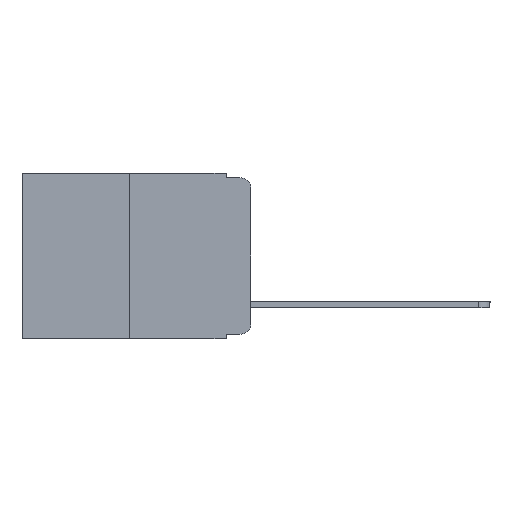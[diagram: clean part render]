
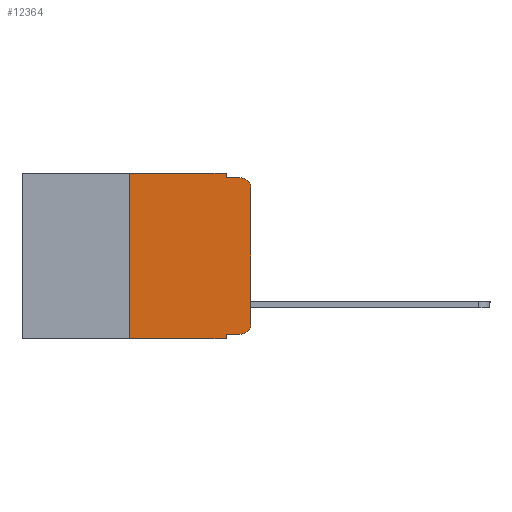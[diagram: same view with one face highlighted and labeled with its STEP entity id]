
A CAD part, left-side view. The second image highlights one B-rep face of the part: STEP entity #12364.
In plain terms, the highlighted planar face has unit normal (-1, 0, 0).
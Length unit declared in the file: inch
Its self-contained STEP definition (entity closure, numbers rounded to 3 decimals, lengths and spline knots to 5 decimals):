
#435 = CARTESIAN_POINT ( 'NONE',  ( 0., 0.051, -0.343 ) ) ;
#567 = EDGE_CURVE ( 'NONE', #7809, #8630, #12805, .T. ) ;
#664 = EDGE_CURVE ( 'NONE', #2239, #8630, #15236, .T. ) ;
#1151 = DIRECTION ( 'NONE',  ( 0., 0., -1. ) ) ;
#1229 = DIRECTION ( 'NONE',  ( 0., -1., 0. ) ) ;
#1307 = CARTESIAN_POINT ( 'NONE',  ( 0., 0.473, -0.343 ) ) ;
#1357 = EDGE_CURVE ( 'NONE', #1494, #16598, #14682, .T. ) ;
#1494 = VERTEX_POINT ( 'NONE', #13778 ) ;
#1995 = LINE ( 'NONE', #6937, #15735 ) ;
#2175 = LINE ( 'NONE', #12326, #12218 ) ;
#2224 = EDGE_CURVE ( 'NONE', #6799, #7569, #5821, .T. ) ;
#2239 = VERTEX_POINT ( 'NONE', #7252 ) ;
#2255 = DIRECTION ( 'NONE',  ( 0., 0., 1. ) ) ;
#2298 = DIRECTION ( 'NONE',  ( 0., -1., 0. ) ) ;
#2672 = VECTOR ( 'NONE', #6170, 39.37008 ) ;
#2776 = LINE ( 'NONE', #7892, #5738 ) ;
#2822 = FACE_OUTER_BOUND ( 'NONE', #13756, .T. ) ;
#3107 = DIRECTION ( 'NONE',  ( -1., 0., 0. ) ) ;
#3503 = CARTESIAN_POINT ( 'NONE',  ( 0., 0.02, -0.01 ) ) ;
#4070 = PLANE ( 'NONE',  #7480 ) ;
#4103 = EDGE_CURVE ( 'NONE', #2239, #13249, #2776, .T. ) ;
#4163 = CARTESIAN_POINT ( 'NONE',  ( 0., 0.02, -0.333 ) ) ;
#4225 = CARTESIAN_POINT ( 'NONE',  ( 0., 0.02, -0.313 ) ) ;
#4467 = CARTESIAN_POINT ( 'NONE',  ( 0., 0.051, 0. ) ) ;
#5010 = CARTESIAN_POINT ( 'NONE',  ( 0., 0.25, 0. ) ) ;
#5288 = CIRCLE ( 'NONE', #10137, 0.02 ) ;
#5408 = CARTESIAN_POINT ( 'NONE',  ( 0., 0.473, 0. ) ) ;
#5446 = DIRECTION ( 'NONE',  ( 0., -1., 0. ) ) ;
#5738 = VECTOR ( 'NONE', #5446, 39.37008 ) ;
#5821 = LINE ( 'NONE', #12205, #15008 ) ;
#5926 = VECTOR ( 'NONE', #7473, 39.37008 ) ;
#6170 = DIRECTION ( 'NONE',  ( 0., 0., -1. ) ) ;
#6266 = CARTESIAN_POINT ( 'NONE',  ( 0., 0.051, 0. ) ) ;
#6791 = EDGE_CURVE ( 'NONE', #7809, #6799, #2175, .T. ) ;
#6799 = VERTEX_POINT ( 'NONE', #5010 ) ;
#6937 = CARTESIAN_POINT ( 'NONE',  ( 0., 0.051, -0.01 ) ) ;
#7252 = CARTESIAN_POINT ( 'NONE',  ( 0., 0.051, -0.333 ) ) ;
#7395 = CARTESIAN_POINT ( 'NONE',  ( 0., 0., -0.313 ) ) ;
#7473 = DIRECTION ( 'NONE',  ( 0., 0., 1. ) ) ;
#7480 = AXIS2_PLACEMENT_3D ( 'NONE', #5408, #9197, #10786 ) ;
#7569 = VERTEX_POINT ( 'NONE', #4467 ) ;
#7628 = ORIENTED_EDGE ( 'NONE', *, *, #1357, .T. ) ;
#7809 = VERTEX_POINT ( 'NONE', #11606 ) ;
#7892 = CARTESIAN_POINT ( 'NONE',  ( 0., 0.051, -0.333 ) ) ;
#7959 = ORIENTED_EDGE ( 'NONE', *, *, #4103, .T. ) ;
#8393 = DIRECTION ( 'NONE',  ( 0., 0., -1. ) ) ;
#8570 = LINE ( 'NONE', #8654, #5926 ) ;
#8624 = ORIENTED_EDGE ( 'NONE', *, *, #14345, .T. ) ;
#8630 = VERTEX_POINT ( 'NONE', #435 ) ;
#8654 = CARTESIAN_POINT ( 'NONE',  ( 0., 0., 0. ) ) ;
#8930 = CARTESIAN_POINT ( 'NONE',  ( 0., 0.051, -0.01 ) ) ;
#9019 = EDGE_CURVE ( 'NONE', #15285, #16598, #1995, .T. ) ;
#9164 = EDGE_CURVE ( 'NONE', #7569, #15285, #15164, .T. ) ;
#9197 = DIRECTION ( 'NONE',  ( 1., 0., 0. ) ) ;
#9323 = AXIS2_PLACEMENT_3D ( 'NONE', #15864, #3107, #8393 ) ;
#9456 = EDGE_CURVE ( 'NONE', #13249, #14450, #5288, .T. ) ;
#9581 = VECTOR ( 'NONE', #1151, 39.37008 ) ;
#9767 = ORIENTED_EDGE ( 'NONE', *, *, #2224, .F. ) ;
#10137 = AXIS2_PLACEMENT_3D ( 'NONE', #4225, #14649, #13307 ) ;
#10786 = DIRECTION ( 'NONE',  ( 0., 0., -1. ) ) ;
#11147 = ORIENTED_EDGE ( 'NONE', *, *, #664, .F. ) ;
#11606 = CARTESIAN_POINT ( 'NONE',  ( 0., 0.25, -0.343 ) ) ;
#12205 = CARTESIAN_POINT ( 'NONE',  ( 0., 0.473, 0. ) ) ;
#12218 = VECTOR ( 'NONE', #2255, 39.37008 ) ;
#12234 = ORIENTED_EDGE ( 'NONE', *, *, #9164, .F. ) ;
#12326 = CARTESIAN_POINT ( 'NONE',  ( 0., 0.25, 0. ) ) ;
#12364 = ADVANCED_FACE ( 'NONE', ( #2822 ), #4070, .F. ) ;
#12548 = CARTESIAN_POINT ( 'NONE',  ( 0., 0.051, 0. ) ) ;
#12558 = ORIENTED_EDGE ( 'NONE', *, *, #567, .T. ) ;
#12805 = LINE ( 'NONE', #1307, #14215 ) ;
#13249 = VERTEX_POINT ( 'NONE', #4163 ) ;
#13307 = DIRECTION ( 'NONE',  ( 0., 0., -1. ) ) ;
#13756 = EDGE_LOOP ( 'NONE', ( #8624, #7628, #14270, #12234, #9767, #15403, #12558, #11147, #7959, #16516 ) ) ;
#13778 = CARTESIAN_POINT ( 'NONE',  ( 0., 0., -0.03 ) ) ;
#14215 = VECTOR ( 'NONE', #1229, 39.37008 ) ;
#14270 = ORIENTED_EDGE ( 'NONE', *, *, #9019, .F. ) ;
#14345 = EDGE_CURVE ( 'NONE', #14450, #1494, #8570, .T. ) ;
#14450 = VERTEX_POINT ( 'NONE', #7395 ) ;
#14649 = DIRECTION ( 'NONE',  ( -1., 0., 0. ) ) ;
#14682 = CIRCLE ( 'NONE', #9323, 0.02 ) ;
#15008 = VECTOR ( 'NONE', #2298, 39.37008 ) ;
#15164 = LINE ( 'NONE', #6266, #9581 ) ;
#15236 = LINE ( 'NONE', #12548, #2672 ) ;
#15285 = VERTEX_POINT ( 'NONE', #8930 ) ;
#15403 = ORIENTED_EDGE ( 'NONE', *, *, #6791, .F. ) ;
#15735 = VECTOR ( 'NONE', #16170, 39.37008 ) ;
#15864 = CARTESIAN_POINT ( 'NONE',  ( 0., 0.02, -0.03 ) ) ;
#16170 = DIRECTION ( 'NONE',  ( 0., -1., 0. ) ) ;
#16516 = ORIENTED_EDGE ( 'NONE', *, *, #9456, .T. ) ;
#16598 = VERTEX_POINT ( 'NONE', #3503 ) ;
